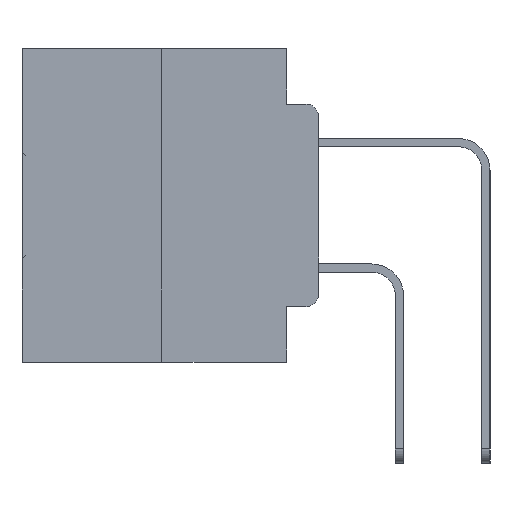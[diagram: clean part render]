
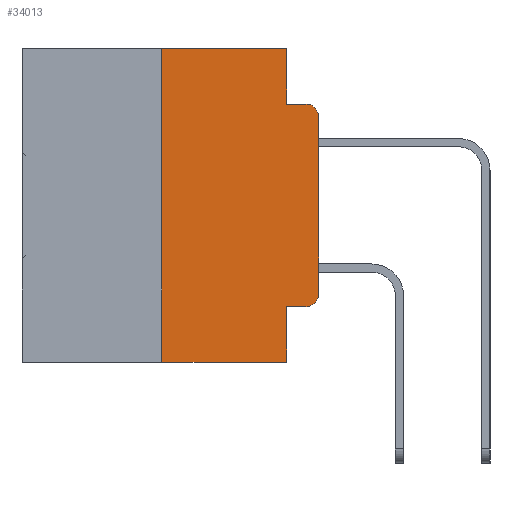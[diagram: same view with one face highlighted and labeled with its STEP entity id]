
A CAD part, left-side view. The second image highlights one B-rep face of the part: STEP entity #34013.
In plain terms, the highlighted planar face has unit normal (-1, 0, 0).
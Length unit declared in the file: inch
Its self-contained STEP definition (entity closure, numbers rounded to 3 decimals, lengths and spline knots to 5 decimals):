
#336 = DIRECTION ( 'NONE',  ( 0., 0., -1. ) ) ;
#516 = ORIENTED_EDGE ( 'NONE', *, *, #23495, .F. ) ;
#961 = CARTESIAN_POINT ( 'NONE',  ( 0., 0.051, -0.4115 ) ) ;
#1136 = CARTESIAN_POINT ( 'NONE',  ( 0., 0.25, -0.5 ) ) ;
#1278 = LINE ( 'NONE', #11036, #12885 ) ;
#1475 = CARTESIAN_POINT ( 'NONE',  ( 0., 0., -0.3915 ) ) ;
#2183 = DIRECTION ( 'NONE',  ( 0., 0., -1. ) ) ;
#2389 = VECTOR ( 'NONE', #7011, 39.37008 ) ;
#3510 = VERTEX_POINT ( 'NONE', #6948 ) ;
#5036 = ORIENTED_EDGE ( 'NONE', *, *, #30736, .T. ) ;
#6676 = ORIENTED_EDGE ( 'NONE', *, *, #23038, .T. ) ;
#6948 = CARTESIAN_POINT ( 'NONE',  ( 0., 0.051, -0.5 ) ) ;
#7011 = DIRECTION ( 'NONE',  ( 0., -1., 0. ) ) ;
#7104 = CIRCLE ( 'NONE', #14151, 0.02 ) ;
#7177 = CARTESIAN_POINT ( 'NONE',  ( 0., 0.473, -0.5 ) ) ;
#8060 = DIRECTION ( 'NONE',  ( 0., -1., 0. ) ) ;
#9365 = EDGE_CURVE ( 'NONE', #18049, #10583, #27024, .T. ) ;
#9853 = VERTEX_POINT ( 'NONE', #1475 ) ;
#10583 = VERTEX_POINT ( 'NONE', #28759 ) ;
#10680 = VERTEX_POINT ( 'NONE', #29098 ) ;
#10973 = VECTOR ( 'NONE', #25837, 39.37008 ) ;
#11036 = CARTESIAN_POINT ( 'NONE',  ( 0., 0.473, 0. ) ) ;
#11483 = DIRECTION ( 'NONE',  ( 0., 0., 1. ) ) ;
#11623 = PLANE ( 'NONE',  #28362 ) ;
#11738 = DIRECTION ( 'NONE',  ( 1., 0., 0. ) ) ;
#12113 = EDGE_CURVE ( 'NONE', #10680, #9853, #7104, .T. ) ;
#12485 = DIRECTION ( 'NONE',  ( -1., 0., 0. ) ) ;
#12575 = ORIENTED_EDGE ( 'NONE', *, *, #27659, .T. ) ;
#12819 = EDGE_CURVE ( 'NONE', #10583, #25580, #1278, .T. ) ;
#12885 = VECTOR ( 'NONE', #16339, 39.37008 ) ;
#12979 = ORIENTED_EDGE ( 'NONE', *, *, #9365, .F. ) ;
#13010 = ORIENTED_EDGE ( 'NONE', *, *, #14853, .F. ) ;
#13080 = VERTEX_POINT ( 'NONE', #26096 ) ;
#13382 = ORIENTED_EDGE ( 'NONE', *, *, #12819, .F. ) ;
#13448 = ORIENTED_EDGE ( 'NONE', *, *, #12113, .T. ) ;
#13955 = LINE ( 'NONE', #26702, #28095 ) ;
#14151 = AXIS2_PLACEMENT_3D ( 'NONE', #32045, #16268, #336 ) ;
#14725 = ORIENTED_EDGE ( 'NONE', *, *, #18202, .T. ) ;
#14853 = EDGE_CURVE ( 'NONE', #15793, #3510, #33393, .T. ) ;
#15474 = CARTESIAN_POINT ( 'NONE',  ( 0., 0.25, 0. ) ) ;
#15793 = VERTEX_POINT ( 'NONE', #961 ) ;
#16268 = DIRECTION ( 'NONE',  ( -1., 0., 0. ) ) ;
#16339 = DIRECTION ( 'NONE',  ( 0., -1., 0. ) ) ;
#16779 = CARTESIAN_POINT ( 'NONE',  ( 0., 0., 0. ) ) ;
#18049 = VERTEX_POINT ( 'NONE', #1136 ) ;
#18202 = EDGE_CURVE ( 'NONE', #15793, #10680, #30587, .T. ) ;
#18287 = LINE ( 'NONE', #16779, #31450 ) ;
#18826 = FACE_OUTER_BOUND ( 'NONE', #30562, .T. ) ;
#19463 = VECTOR ( 'NONE', #2183, 39.37008 ) ;
#19715 = CARTESIAN_POINT ( 'NONE',  ( 0., 0.473, 0. ) ) ;
#20202 = DIRECTION ( 'NONE',  ( 0., 0., -1. ) ) ;
#20488 = ORIENTED_EDGE ( 'NONE', *, *, #26595, .F. ) ;
#22437 = VERTEX_POINT ( 'NONE', #25940 ) ;
#23038 = EDGE_CURVE ( 'NONE', #25942, #13080, #30301, .T. ) ;
#23495 = EDGE_CURVE ( 'NONE', #25580, #22437, #33555, .T. ) ;
#23733 = CARTESIAN_POINT ( 'NONE',  ( 0., 0., -0.1085 ) ) ;
#25580 = VERTEX_POINT ( 'NONE', #27809 ) ;
#25837 = DIRECTION ( 'NONE',  ( 0., -1., 0. ) ) ;
#25940 = CARTESIAN_POINT ( 'NONE',  ( 0., 0.051, -0.0885 ) ) ;
#25942 = VERTEX_POINT ( 'NONE', #23733 ) ;
#26096 = CARTESIAN_POINT ( 'NONE',  ( 0., 0.02, -0.0885 ) ) ;
#26595 = EDGE_CURVE ( 'NONE', #22437, #13080, #13955, .T. ) ;
#26667 = VECTOR ( 'NONE', #20202, 39.37008 ) ;
#26702 = CARTESIAN_POINT ( 'NONE',  ( 0., 0.051, -0.0885 ) ) ;
#27024 = LINE ( 'NONE', #15474, #33118 ) ;
#27659 = EDGE_CURVE ( 'NONE', #18049, #3510, #32117, .T. ) ;
#27809 = CARTESIAN_POINT ( 'NONE',  ( 0., 0.051, 0. ) ) ;
#28095 = VECTOR ( 'NONE', #8060, 39.37008 ) ;
#28194 = CARTESIAN_POINT ( 'NONE',  ( 0., 0.051, -0.4115 ) ) ;
#28196 = AXIS2_PLACEMENT_3D ( 'NONE', #28431, #12485, #31030 ) ;
#28362 = AXIS2_PLACEMENT_3D ( 'NONE', #19715, #11738, #30295 ) ;
#28431 = CARTESIAN_POINT ( 'NONE',  ( 0., 0.02, -0.1085 ) ) ;
#28759 = CARTESIAN_POINT ( 'NONE',  ( 0., 0.25, 0. ) ) ;
#29098 = CARTESIAN_POINT ( 'NONE',  ( 0., 0.02, -0.4115 ) ) ;
#30295 = DIRECTION ( 'NONE',  ( 0., 0., -1. ) ) ;
#30301 = CIRCLE ( 'NONE', #28196, 0.02 ) ;
#30562 = EDGE_LOOP ( 'NONE', ( #5036, #6676, #20488, #516, #13382, #12979, #12575, #13010, #14725, #13448 ) ) ;
#30587 = LINE ( 'NONE', #28194, #2389 ) ;
#30663 = CARTESIAN_POINT ( 'NONE',  ( 0., 0.051, 0. ) ) ;
#30736 = EDGE_CURVE ( 'NONE', #9853, #25942, #18287, .T. ) ;
#31030 = DIRECTION ( 'NONE',  ( 0., 0., -1. ) ) ;
#31450 = VECTOR ( 'NONE', #11483, 39.37008 ) ;
#32045 = CARTESIAN_POINT ( 'NONE',  ( 0., 0.02, -0.3915 ) ) ;
#32117 = LINE ( 'NONE', #7177, #10973 ) ;
#33118 = VECTOR ( 'NONE', #33860, 39.37008 ) ;
#33393 = LINE ( 'NONE', #33828, #19463 ) ;
#33555 = LINE ( 'NONE', #30663, #26667 ) ;
#33828 = CARTESIAN_POINT ( 'NONE',  ( 0., 0.051, 0. ) ) ;
#33860 = DIRECTION ( 'NONE',  ( 0., 0., 1. ) ) ;
#34013 = ADVANCED_FACE ( 'NONE', ( #18826 ), #11623, .F. ) ;
